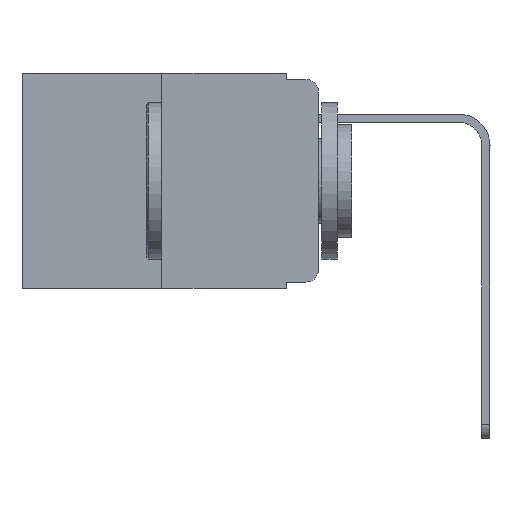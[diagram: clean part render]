
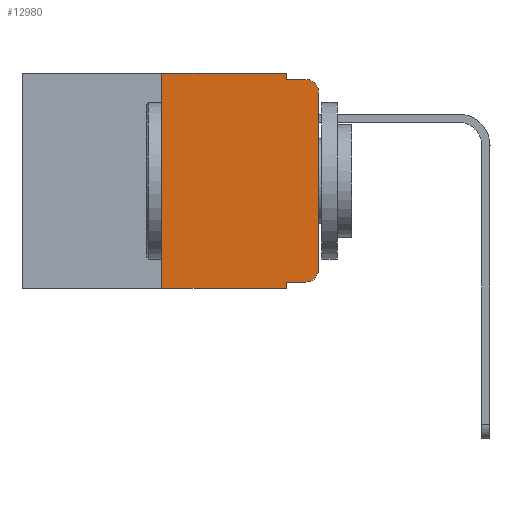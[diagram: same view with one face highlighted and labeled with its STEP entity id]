
A CAD part, left-side view. The second image highlights one B-rep face of the part: STEP entity #12980.
In plain terms, the highlighted planar face has unit normal (-1, 0, 0).
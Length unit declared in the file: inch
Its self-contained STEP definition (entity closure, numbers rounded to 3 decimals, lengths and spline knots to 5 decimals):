
#94 = ORIENTED_EDGE ( 'NONE', *, *, #14152, .F. ) ;
#116 = VECTOR ( 'NONE', #11165, 39.37008 ) ;
#327 = CARTESIAN_POINT ( 'NONE',  ( 0., 0.25, 0. ) ) ;
#344 = CIRCLE ( 'NONE', #9761, 0.02 ) ;
#463 = VERTEX_POINT ( 'NONE', #3992 ) ;
#477 = VECTOR ( 'NONE', #7030, 39.37008 ) ;
#531 = CARTESIAN_POINT ( 'NONE',  ( 0., 0.051, 0. ) ) ;
#698 = AXIS2_PLACEMENT_3D ( 'NONE', #11783, #14128, #5998 ) ;
#725 = LINE ( 'NONE', #13608, #4410 ) ;
#851 = LINE ( 'NONE', #10204, #116 ) ;
#1076 = DIRECTION ( 'NONE',  ( 1., 0., 0. ) ) ;
#1322 = CARTESIAN_POINT ( 'NONE',  ( 0., 0., -0.03 ) ) ;
#2196 = EDGE_CURVE ( 'NONE', #10058, #8664, #7207, .T. ) ;
#2303 = DIRECTION ( 'NONE',  ( 0., -1., 0. ) ) ;
#2359 = VERTEX_POINT ( 'NONE', #6410 ) ;
#2360 = VECTOR ( 'NONE', #4131, 39.37008 ) ;
#2513 = ORIENTED_EDGE ( 'NONE', *, *, #10238, .F. ) ;
#2521 = VERTEX_POINT ( 'NONE', #10195 ) ;
#2890 = LINE ( 'NONE', #12763, #8250 ) ;
#2908 = VECTOR ( 'NONE', #13908, 39.37008 ) ;
#3047 = ORIENTED_EDGE ( 'NONE', *, *, #12384, .T. ) ;
#3456 = CARTESIAN_POINT ( 'NONE',  ( 0., 0.051, -0.01 ) ) ;
#3800 = VERTEX_POINT ( 'NONE', #4216 ) ;
#3992 = CARTESIAN_POINT ( 'NONE',  ( 0., 0.25, -0.343 ) ) ;
#4131 = DIRECTION ( 'NONE',  ( 0., 0., -1. ) ) ;
#4167 = DIRECTION ( 'NONE',  ( 0., 0., -1. ) ) ;
#4216 = CARTESIAN_POINT ( 'NONE',  ( 0., 0.051, -0.343 ) ) ;
#4297 = ORIENTED_EDGE ( 'NONE', *, *, #13093, .T. ) ;
#4410 = VECTOR ( 'NONE', #4167, 39.37008 ) ;
#4736 = CARTESIAN_POINT ( 'NONE',  ( 0., 0.473, 0. ) ) ;
#4783 = AXIS2_PLACEMENT_3D ( 'NONE', #4736, #1076, #5675 ) ;
#5107 = FACE_OUTER_BOUND ( 'NONE', #7970, .T. ) ;
#5675 = DIRECTION ( 'NONE',  ( 0., 0., -1. ) ) ;
#5875 = VECTOR ( 'NONE', #15045, 39.37008 ) ;
#5998 = DIRECTION ( 'NONE',  ( 0., 0., -1. ) ) ;
#6218 = ORIENTED_EDGE ( 'NONE', *, *, #12943, .T. ) ;
#6410 = CARTESIAN_POINT ( 'NONE',  ( 0., 0.051, -0.333 ) ) ;
#7030 = DIRECTION ( 'NONE',  ( 0., -1., 0. ) ) ;
#7207 = CIRCLE ( 'NONE', #698, 0.02 ) ;
#7310 = DIRECTION ( 'NONE',  ( 0., -1., 0. ) ) ;
#7485 = LINE ( 'NONE', #3456, #477 ) ;
#7881 = EDGE_CURVE ( 'NONE', #2359, #3800, #725, .T. ) ;
#7970 = EDGE_LOOP ( 'NONE', ( #3047, #13873, #94, #2513, #10763, #13538, #6218, #9224, #4297, #12149 ) ) ;
#8064 = VERTEX_POINT ( 'NONE', #11662 ) ;
#8250 = VECTOR ( 'NONE', #2303, 39.37008 ) ;
#8621 = DIRECTION ( 'NONE',  ( -1., 0., 0. ) ) ;
#8664 = VERTEX_POINT ( 'NONE', #12839 ) ;
#8982 = VERTEX_POINT ( 'NONE', #14605 ) ;
#9224 = ORIENTED_EDGE ( 'NONE', *, *, #7881, .F. ) ;
#9761 = AXIS2_PLACEMENT_3D ( 'NONE', #9801, #8621, #14480 ) ;
#9801 = CARTESIAN_POINT ( 'NONE',  ( 0., 0.02, -0.313 ) ) ;
#10053 = EDGE_CURVE ( 'NONE', #8064, #12365, #344, .T. ) ;
#10058 = VERTEX_POINT ( 'NONE', #1322 ) ;
#10087 = LINE ( 'NONE', #14294, #14096 ) ;
#10195 = CARTESIAN_POINT ( 'NONE',  ( 0., 0.051, -0.01 ) ) ;
#10204 = CARTESIAN_POINT ( 'NONE',  ( 0., 0.25, 0. ) ) ;
#10238 = EDGE_CURVE ( 'NONE', #8982, #2521, #13938, .T. ) ;
#10386 = CARTESIAN_POINT ( 'NONE',  ( 0., 0.473, 0. ) ) ;
#10667 = LINE ( 'NONE', #12820, #2908 ) ;
#10763 = ORIENTED_EDGE ( 'NONE', *, *, #12994, .F. ) ;
#10766 = VERTEX_POINT ( 'NONE', #327 ) ;
#11165 = DIRECTION ( 'NONE',  ( 0., 0., 1. ) ) ;
#11662 = CARTESIAN_POINT ( 'NONE',  ( 0., 0.02, -0.333 ) ) ;
#11707 = CARTESIAN_POINT ( 'NONE',  ( 0., 0., -0.313 ) ) ;
#11755 = PLANE ( 'NONE',  #4783 ) ;
#11783 = CARTESIAN_POINT ( 'NONE',  ( 0., 0.02, -0.03 ) ) ;
#12149 = ORIENTED_EDGE ( 'NONE', *, *, #10053, .T. ) ;
#12365 = VERTEX_POINT ( 'NONE', #11707 ) ;
#12384 = EDGE_CURVE ( 'NONE', #12365, #10058, #10667, .T. ) ;
#12763 = CARTESIAN_POINT ( 'NONE',  ( 0., 0.473, -0.343 ) ) ;
#12820 = CARTESIAN_POINT ( 'NONE',  ( 0., 0., 0. ) ) ;
#12839 = CARTESIAN_POINT ( 'NONE',  ( 0., 0.02, -0.01 ) ) ;
#12943 = EDGE_CURVE ( 'NONE', #463, #3800, #2890, .T. ) ;
#12980 = ADVANCED_FACE ( 'NONE', ( #5107 ), #11755, .F. ) ;
#12994 = EDGE_CURVE ( 'NONE', #10766, #8982, #13029, .T. ) ;
#13029 = LINE ( 'NONE', #10386, #5875 ) ;
#13093 = EDGE_CURVE ( 'NONE', #2359, #8064, #10087, .T. ) ;
#13538 = ORIENTED_EDGE ( 'NONE', *, *, #13862, .F. ) ;
#13608 = CARTESIAN_POINT ( 'NONE',  ( 0., 0.051, 0. ) ) ;
#13862 = EDGE_CURVE ( 'NONE', #463, #10766, #851, .T. ) ;
#13873 = ORIENTED_EDGE ( 'NONE', *, *, #2196, .T. ) ;
#13908 = DIRECTION ( 'NONE',  ( 0., 0., 1. ) ) ;
#13938 = LINE ( 'NONE', #531, #2360 ) ;
#14096 = VECTOR ( 'NONE', #7310, 39.37008 ) ;
#14128 = DIRECTION ( 'NONE',  ( -1., 0., 0. ) ) ;
#14152 = EDGE_CURVE ( 'NONE', #2521, #8664, #7485, .T. ) ;
#14294 = CARTESIAN_POINT ( 'NONE',  ( 0., 0.051, -0.333 ) ) ;
#14480 = DIRECTION ( 'NONE',  ( 0., 0., -1. ) ) ;
#14605 = CARTESIAN_POINT ( 'NONE',  ( 0., 0.051, 0. ) ) ;
#15045 = DIRECTION ( 'NONE',  ( 0., -1., 0. ) ) ;
